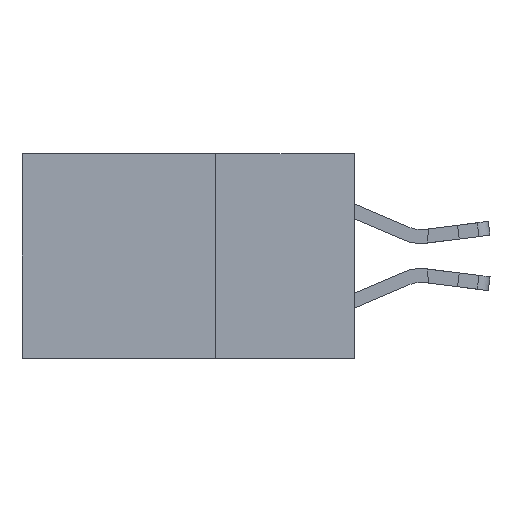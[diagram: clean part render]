
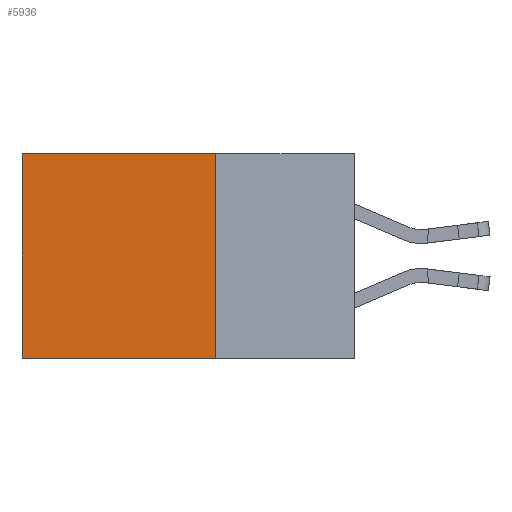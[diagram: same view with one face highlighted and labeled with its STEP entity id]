
A CAD part, left-side view. The second image highlights one B-rep face of the part: STEP entity #5936.
In plain terms, the highlighted planar face has unit normal (-1, 0, 0).
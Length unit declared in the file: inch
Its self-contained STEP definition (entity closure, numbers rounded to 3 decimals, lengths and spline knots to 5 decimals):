
#576 = ORIENTED_EDGE ( 'NONE', *, *, #18794, .F. ) ;
#666 = VECTOR ( 'NONE', #14696, 39.37008 ) ;
#1603 = PLANE ( 'NONE',  #16328 ) ;
#2308 = LINE ( 'NONE', #12776, #17168 ) ;
#2964 = CARTESIAN_POINT ( 'NONE',  ( 0.298, 0.6, 0. ) ) ;
#3115 = DIRECTION ( 'NONE',  ( 1., 0., 0. ) ) ;
#3433 = ORIENTED_EDGE ( 'NONE', *, *, #18842, .F. ) ;
#3917 = CARTESIAN_POINT ( 'NONE',  ( 0.298, 0.25, -0.37 ) ) ;
#4759 = CARTESIAN_POINT ( 'NONE',  ( 0.298, 0.6, 0. ) ) ;
#5532 = LINE ( 'NONE', #4759, #11781 ) ;
#5827 = LINE ( 'NONE', #13378, #666 ) ;
#5936 = ADVANCED_FACE ( 'NONE', ( #14572 ), #1603, .F. ) ;
#6072 = CARTESIAN_POINT ( 'NONE',  ( 0.298, 0.25, 0. ) ) ;
#6549 = VERTEX_POINT ( 'NONE', #3917 ) ;
#6713 = VERTEX_POINT ( 'NONE', #17917 ) ;
#9257 = CARTESIAN_POINT ( 'NONE',  ( 0.298, 0.25, 0. ) ) ;
#9597 = EDGE_LOOP ( 'NONE', ( #10876, #3433, #576, #11038 ) ) ;
#9877 = VERTEX_POINT ( 'NONE', #2964 ) ;
#10030 = DIRECTION ( 'NONE',  ( 0., 0., -1. ) ) ;
#10876 = ORIENTED_EDGE ( 'NONE', *, *, #17246, .T. ) ;
#11038 = ORIENTED_EDGE ( 'NONE', *, *, #16172, .T. ) ;
#11428 = DIRECTION ( 'NONE',  ( 0., 1., 0. ) ) ;
#11781 = VECTOR ( 'NONE', #15145, 39.37008 ) ;
#12776 = CARTESIAN_POINT ( 'NONE',  ( 0.298, 0.25, -0.37 ) ) ;
#13378 = CARTESIAN_POINT ( 'NONE',  ( 0.298, 0.25, 0. ) ) ;
#13479 = DIRECTION ( 'NONE',  ( 0., 0., -1. ) ) ;
#14218 = CARTESIAN_POINT ( 'NONE',  ( 0.298, 0.25, 0. ) ) ;
#14572 = FACE_OUTER_BOUND ( 'NONE', #9597, .T. ) ;
#14696 = DIRECTION ( 'NONE',  ( 0., 1., 0. ) ) ;
#15145 = DIRECTION ( 'NONE',  ( 0., 0., -1. ) ) ;
#15576 = VECTOR ( 'NONE', #10030, 39.37008 ) ;
#16172 = EDGE_CURVE ( 'NONE', #16279, #9877, #5827, .T. ) ;
#16279 = VERTEX_POINT ( 'NONE', #9257 ) ;
#16328 = AXIS2_PLACEMENT_3D ( 'NONE', #6072, #3115, #13479 ) ;
#17168 = VECTOR ( 'NONE', #11428, 39.37008 ) ;
#17246 = EDGE_CURVE ( 'NONE', #9877, #6713, #5532, .T. ) ;
#17646 = LINE ( 'NONE', #14218, #15576 ) ;
#17917 = CARTESIAN_POINT ( 'NONE',  ( 0.298, 0.6, -0.37 ) ) ;
#18794 = EDGE_CURVE ( 'NONE', #16279, #6549, #17646, .T. ) ;
#18842 = EDGE_CURVE ( 'NONE', #6549, #6713, #2308, .T. ) ;
